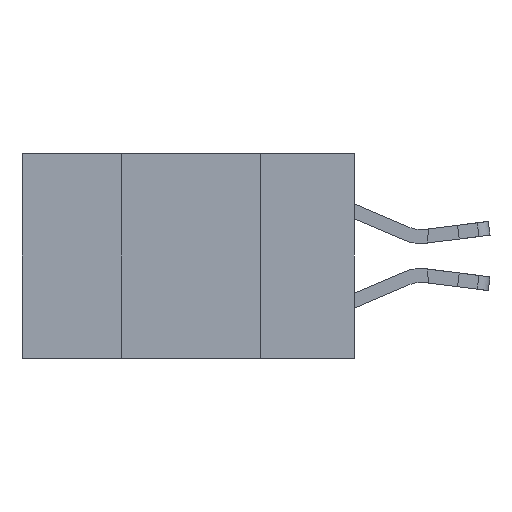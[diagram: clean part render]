
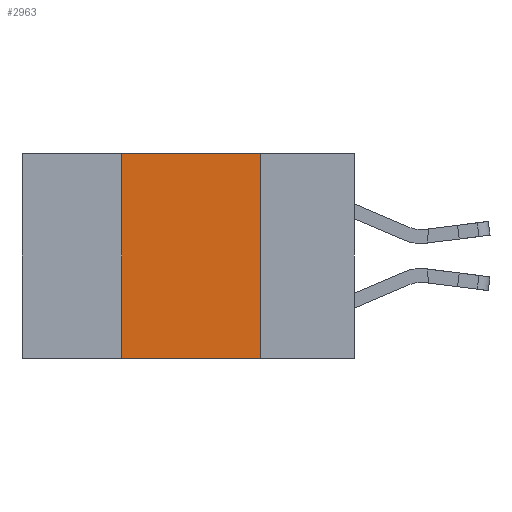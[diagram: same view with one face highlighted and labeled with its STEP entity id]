
A CAD part, left-side view. The second image highlights one B-rep face of the part: STEP entity #2963.
In plain terms, the highlighted planar face has unit normal (-1, 0, 0).
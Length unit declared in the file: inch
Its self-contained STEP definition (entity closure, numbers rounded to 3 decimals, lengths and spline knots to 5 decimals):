
#184 = FACE_OUTER_BOUND ( 'NONE', #12860, .T. ) ;
#711 = CARTESIAN_POINT ( 'NONE',  ( 0., 0.42, -0.37 ) ) ;
#1168 = AXIS2_PLACEMENT_3D ( 'NONE', #17341, #6752, #5266 ) ;
#1580 = CARTESIAN_POINT ( 'NONE',  ( 0., 0.42, 0. ) ) ;
#2813 = LINE ( 'NONE', #4969, #6987 ) ;
#2963 = ADVANCED_FACE ( 'NONE', ( #184 ), #15530, .F. ) ;
#3177 = EDGE_CURVE ( 'NONE', #7244, #21850, #6500, .T. ) ;
#3411 = LINE ( 'NONE', #20487, #15614 ) ;
#3619 = EDGE_CURVE ( 'NONE', #21228, #7244, #2813, .T. ) ;
#4451 = DIRECTION ( 'NONE',  ( 0., 0., 1. ) ) ;
#4969 = CARTESIAN_POINT ( 'NONE',  ( 0., 0.6, 0. ) ) ;
#5266 = DIRECTION ( 'NONE',  ( 0., 0., -1. ) ) ;
#6500 = LINE ( 'NONE', #21543, #17074 ) ;
#6752 = DIRECTION ( 'NONE',  ( 1., 0., 0. ) ) ;
#6987 = VECTOR ( 'NONE', #20467, 39.37008 ) ;
#7244 = VERTEX_POINT ( 'NONE', #21918 ) ;
#8794 = CARTESIAN_POINT ( 'NONE',  ( 0., 0.42, -0.37 ) ) ;
#10012 = ORIENTED_EDGE ( 'NONE', *, *, #13797, .F. ) ;
#11583 = CARTESIAN_POINT ( 'NONE',  ( 0., 0.17, -0.37 ) ) ;
#12860 = EDGE_LOOP ( 'NONE', ( #16172, #17933, #10012, #15054 ) ) ;
#12883 = EDGE_CURVE ( 'NONE', #16657, #21850, #3411, .T. ) ;
#13267 = DIRECTION ( 'NONE',  ( 0., 0., -1. ) ) ;
#13797 = EDGE_CURVE ( 'NONE', #16657, #21228, #21637, .T. ) ;
#15054 = ORIENTED_EDGE ( 'NONE', *, *, #12883, .T. ) ;
#15530 = PLANE ( 'NONE',  #1168 ) ;
#15614 = VECTOR ( 'NONE', #18890, 39.37008 ) ;
#16172 = ORIENTED_EDGE ( 'NONE', *, *, #3177, .F. ) ;
#16657 = VERTEX_POINT ( 'NONE', #8794 ) ;
#17074 = VECTOR ( 'NONE', #13267, 39.37008 ) ;
#17341 = CARTESIAN_POINT ( 'NONE',  ( 0., 0.6, 0. ) ) ;
#17650 = VECTOR ( 'NONE', #4451, 39.37008 ) ;
#17933 = ORIENTED_EDGE ( 'NONE', *, *, #3619, .F. ) ;
#18890 = DIRECTION ( 'NONE',  ( 0., -1., 0. ) ) ;
#20467 = DIRECTION ( 'NONE',  ( 0., -1., 0. ) ) ;
#20487 = CARTESIAN_POINT ( 'NONE',  ( 0., 0.6, -0.37 ) ) ;
#21228 = VERTEX_POINT ( 'NONE', #1580 ) ;
#21543 = CARTESIAN_POINT ( 'NONE',  ( 0., 0.17, -0.37 ) ) ;
#21637 = LINE ( 'NONE', #711, #17650 ) ;
#21850 = VERTEX_POINT ( 'NONE', #11583 ) ;
#21918 = CARTESIAN_POINT ( 'NONE',  ( 0., 0.17, 0. ) ) ;
